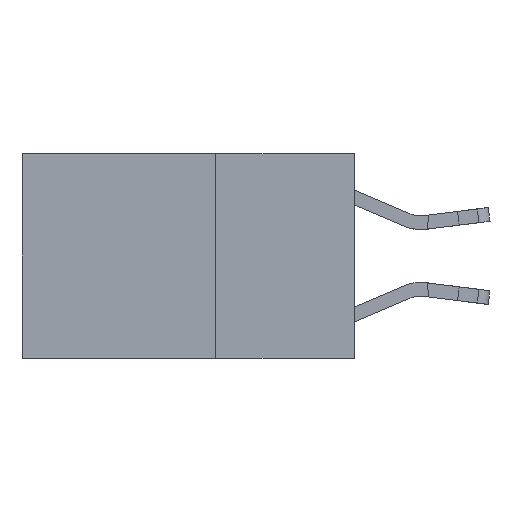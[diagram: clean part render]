
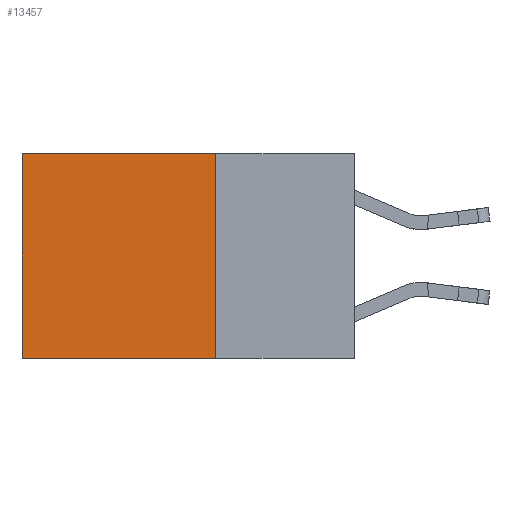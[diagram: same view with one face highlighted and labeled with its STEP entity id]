
A CAD part, left-side view. The second image highlights one B-rep face of the part: STEP entity #13457.
In plain terms, the highlighted planar face has unit normal (-1, 0, 0).
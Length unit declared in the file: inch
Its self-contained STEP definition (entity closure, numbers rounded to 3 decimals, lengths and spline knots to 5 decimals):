
#231 = VERTEX_POINT ( 'NONE', #11510 ) ;
#582 = DIRECTION ( 'NONE',  ( 1., 0., 0. ) ) ;
#1116 = CARTESIAN_POINT ( 'NONE',  ( 0.2625, 0.25, -0.37 ) ) ;
#1300 = ORIENTED_EDGE ( 'NONE', *, *, #13130, .T. ) ;
#1902 = EDGE_CURVE ( 'NONE', #231, #17089, #3933, .T. ) ;
#1943 = DIRECTION ( 'NONE',  ( 0., 0., -1. ) ) ;
#2532 = DIRECTION ( 'NONE',  ( 0., 1., 0. ) ) ;
#2567 = CARTESIAN_POINT ( 'NONE',  ( 0.2625, 0.25, 0. ) ) ;
#2569 = DIRECTION ( 'NONE',  ( 0., 0., -1. ) ) ;
#3933 = LINE ( 'NONE', #10252, #10878 ) ;
#4218 = EDGE_CURVE ( 'NONE', #17089, #16579, #16619, .T. ) ;
#5135 = CARTESIAN_POINT ( 'NONE',  ( 0.2625, 0.6, -0.37 ) ) ;
#5244 = EDGE_CURVE ( 'NONE', #6178, #16579, #12307, .T. ) ;
#5418 = ORIENTED_EDGE ( 'NONE', *, *, #5244, .T. ) ;
#5660 = CARTESIAN_POINT ( 'NONE',  ( 0.2625, 0.6, 0. ) ) ;
#5853 = AXIS2_PLACEMENT_3D ( 'NONE', #7534, #582, #10334 ) ;
#6178 = VERTEX_POINT ( 'NONE', #5660 ) ;
#6387 = LINE ( 'NONE', #2567, #16954 ) ;
#6709 = CARTESIAN_POINT ( 'NONE',  ( 0.2625, 0.6, 0. ) ) ;
#7239 = FACE_OUTER_BOUND ( 'NONE', #14248, .T. ) ;
#7489 = CARTESIAN_POINT ( 'NONE',  ( 0.2625, 0.25, -0.37 ) ) ;
#7534 = CARTESIAN_POINT ( 'NONE',  ( 0.2625, 0.25, 0. ) ) ;
#8710 = ORIENTED_EDGE ( 'NONE', *, *, #4218, .F. ) ;
#9484 = DIRECTION ( 'NONE',  ( 0., 1., 0. ) ) ;
#10252 = CARTESIAN_POINT ( 'NONE',  ( 0.2625, 0.25, 0. ) ) ;
#10334 = DIRECTION ( 'NONE',  ( 0., 0., -1. ) ) ;
#10878 = VECTOR ( 'NONE', #1943, 39.37008 ) ;
#11510 = CARTESIAN_POINT ( 'NONE',  ( 0.2625, 0.25, 0. ) ) ;
#12307 = LINE ( 'NONE', #6709, #16001 ) ;
#12962 = VECTOR ( 'NONE', #2532, 39.37008 ) ;
#13130 = EDGE_CURVE ( 'NONE', #231, #6178, #6387, .T. ) ;
#13457 = ADVANCED_FACE ( 'NONE', ( #7239 ), #17190, .F. ) ;
#14248 = EDGE_LOOP ( 'NONE', ( #5418, #8710, #16673, #1300 ) ) ;
#16001 = VECTOR ( 'NONE', #2569, 39.37008 ) ;
#16579 = VERTEX_POINT ( 'NONE', #5135 ) ;
#16619 = LINE ( 'NONE', #1116, #12962 ) ;
#16673 = ORIENTED_EDGE ( 'NONE', *, *, #1902, .F. ) ;
#16954 = VECTOR ( 'NONE', #9484, 39.37008 ) ;
#17089 = VERTEX_POINT ( 'NONE', #7489 ) ;
#17190 = PLANE ( 'NONE',  #5853 ) ;
